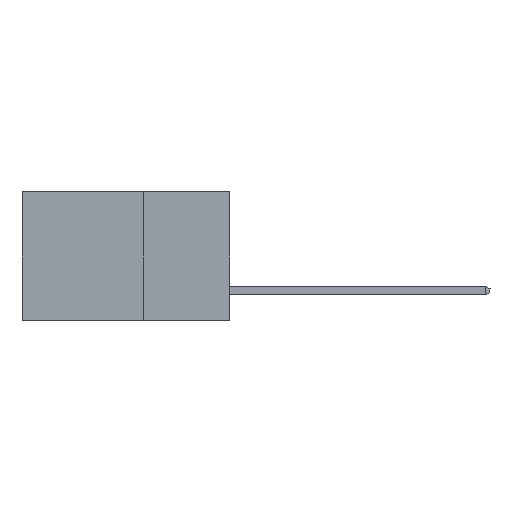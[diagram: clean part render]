
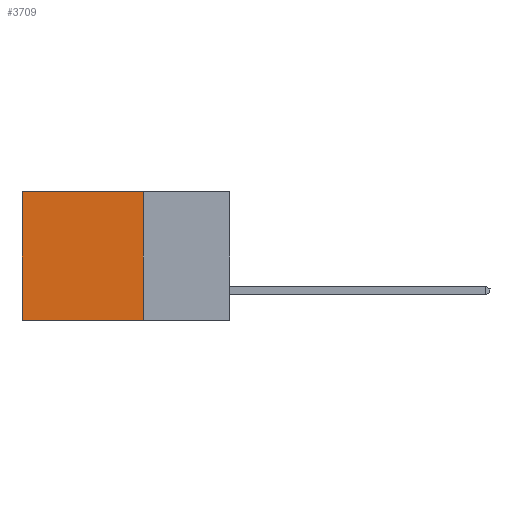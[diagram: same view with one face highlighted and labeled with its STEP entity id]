
A CAD part, left-side view. The second image highlights one B-rep face of the part: STEP entity #3709.
In plain terms, the highlighted planar face has unit normal (-1, 0, 0).
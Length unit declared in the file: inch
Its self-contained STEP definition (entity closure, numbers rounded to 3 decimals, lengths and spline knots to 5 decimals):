
#25 = LINE ( 'NONE', #6873, #3086 ) ;
#200 = LINE ( 'NONE', #12255, #5081 ) ;
#1400 = VERTEX_POINT ( 'NONE', #3594 ) ;
#1780 = EDGE_CURVE ( 'NONE', #1400, #6281, #5555, .T. ) ;
#2215 = LINE ( 'NONE', #4164, #12377 ) ;
#2568 = AXIS2_PLACEMENT_3D ( 'NONE', #4512, #3666, #6496 ) ;
#2593 = DIRECTION ( 'NONE',  ( 0., 1., 0. ) ) ;
#3086 = VECTOR ( 'NONE', #4882, 39.37008 ) ;
#3594 = CARTESIAN_POINT ( 'NONE',  ( 0.2615, 0.25, -0.37 ) ) ;
#3666 = DIRECTION ( 'NONE',  ( 1., 0., 0. ) ) ;
#3709 = ADVANCED_FACE ( 'NONE', ( #8644 ), #10474, .F. ) ;
#4164 = CARTESIAN_POINT ( 'NONE',  ( 0.2615, 0.25, 0. ) ) ;
#4187 = DIRECTION ( 'NONE',  ( 0., 0., -1. ) ) ;
#4512 = CARTESIAN_POINT ( 'NONE',  ( 0.2615, 0.25, -0.37 ) ) ;
#4882 = DIRECTION ( 'NONE',  ( 0., 0., -1. ) ) ;
#5081 = VECTOR ( 'NONE', #4187, 39.37008 ) ;
#5555 = LINE ( 'NONE', #5745, #9512 ) ;
#5603 = ORIENTED_EDGE ( 'NONE', *, *, #9945, .T. ) ;
#5745 = CARTESIAN_POINT ( 'NONE',  ( 0.2615, 0.25, -0.37 ) ) ;
#6281 = VERTEX_POINT ( 'NONE', #7952 ) ;
#6496 = DIRECTION ( 'NONE',  ( 0., 0., -1. ) ) ;
#6497 = VERTEX_POINT ( 'NONE', #6504 ) ;
#6504 = CARTESIAN_POINT ( 'NONE',  ( 0.2615, 0.25, 0. ) ) ;
#6873 = CARTESIAN_POINT ( 'NONE',  ( 0.2615, 0.25, -0.37 ) ) ;
#6952 = ORIENTED_EDGE ( 'NONE', *, *, #1780, .F. ) ;
#7079 = EDGE_LOOP ( 'NONE', ( #7652, #6952, #10973, #5603 ) ) ;
#7106 = EDGE_CURVE ( 'NONE', #6497, #1400, #25, .T. ) ;
#7652 = ORIENTED_EDGE ( 'NONE', *, *, #11022, .T. ) ;
#7952 = CARTESIAN_POINT ( 'NONE',  ( 0.2615, 0.6, -0.37 ) ) ;
#8334 = CARTESIAN_POINT ( 'NONE',  ( 0.2615, 0.6, 0. ) ) ;
#8644 = FACE_OUTER_BOUND ( 'NONE', #7079, .T. ) ;
#9064 = VERTEX_POINT ( 'NONE', #8334 ) ;
#9512 = VECTOR ( 'NONE', #2593, 39.37008 ) ;
#9945 = EDGE_CURVE ( 'NONE', #6497, #9064, #2215, .T. ) ;
#10008 = DIRECTION ( 'NONE',  ( 0., 1., 0. ) ) ;
#10474 = PLANE ( 'NONE',  #2568 ) ;
#10973 = ORIENTED_EDGE ( 'NONE', *, *, #7106, .F. ) ;
#11022 = EDGE_CURVE ( 'NONE', #9064, #6281, #200, .T. ) ;
#12255 = CARTESIAN_POINT ( 'NONE',  ( 0.2615, 0.6, -0.37 ) ) ;
#12377 = VECTOR ( 'NONE', #10008, 39.37008 ) ;
